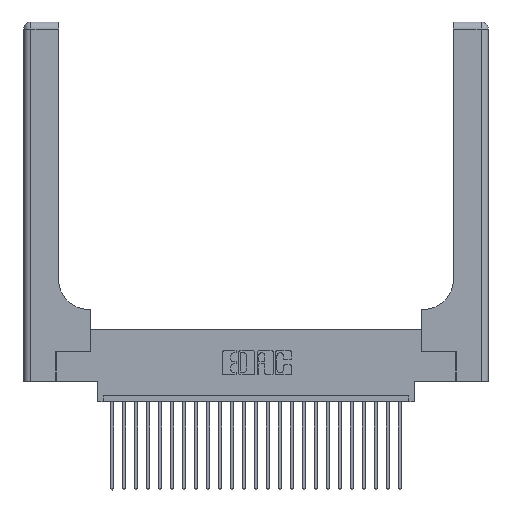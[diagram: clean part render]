
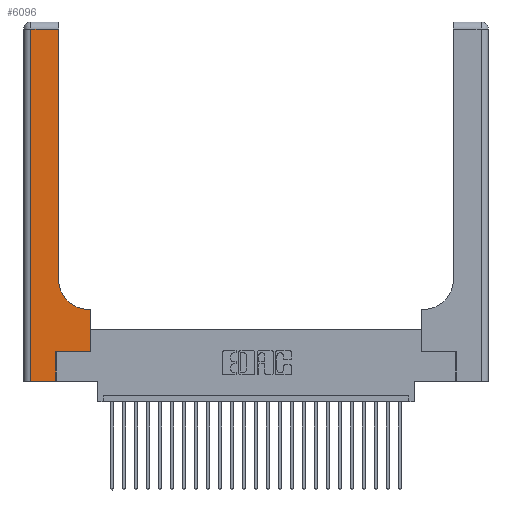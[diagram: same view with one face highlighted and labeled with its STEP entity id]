
A CAD part, top view. The second image highlights one B-rep face of the part: STEP entity #6096.
In plain terms, the highlighted planar face has unit normal (0, 0, 1).
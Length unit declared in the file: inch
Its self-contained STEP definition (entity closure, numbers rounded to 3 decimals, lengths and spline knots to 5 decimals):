
#202 = CARTESIAN_POINT ( 'NONE',  ( 0.269, 0.25, 0.37 ) ) ;
#352 = CARTESIAN_POINT ( 'NONE',  ( 0.2915, 0.6, 0.37 ) ) ;
#2135 = DIRECTION ( 'NONE',  ( -1., 0., 0. ) ) ;
#2240 = DIRECTION ( 'NONE',  ( 1., 0., 0. ) ) ;
#2931 = DIRECTION ( 'NONE',  ( 0., 1., 0. ) ) ;
#3102 = CARTESIAN_POINT ( 'NONE',  ( 0.269, 0., 0.37 ) ) ;
#3140 = EDGE_CURVE ( 'NONE', #15892, #25523, #5019, .T. ) ;
#3253 = DIRECTION ( 'NONE',  ( 0., 1., 0. ) ) ;
#4117 = VERTEX_POINT ( 'NONE', #5091 ) ;
#4272 = EDGE_CURVE ( 'NONE', #12906, #7709, #6530, .T. ) ;
#4456 = CARTESIAN_POINT ( 'NONE',  ( 0.5415, 0.85, 0.37 ) ) ;
#5019 = LINE ( 'NONE', #15736, #18499 ) ;
#5091 = CARTESIAN_POINT ( 'NONE',  ( 0.06, 2.94, 0.37 ) ) ;
#5233 = VECTOR ( 'NONE', #12712, 39.37008 ) ;
#5398 = LINE ( 'NONE', #202, #12792 ) ;
#5425 = EDGE_CURVE ( 'NONE', #25523, #17110, #17441, .T. ) ;
#5749 = DIRECTION ( 'NONE',  ( 0., 1., 0. ) ) ;
#5812 = ORIENTED_EDGE ( 'NONE', *, *, #4272, .T. ) ;
#6096 = ADVANCED_FACE ( 'NONE', ( #8397 ), #20490, .F. ) ;
#6505 = ORIENTED_EDGE ( 'NONE', *, *, #19280, .T. ) ;
#6530 = LINE ( 'NONE', #3102, #16541 ) ;
#6579 = EDGE_CURVE ( 'NONE', #17346, #4117, #7742, .T. ) ;
#6978 = EDGE_CURVE ( 'NONE', #4117, #7243, #22437, .T. ) ;
#7023 = AXIS2_PLACEMENT_3D ( 'NONE', #16443, #26383, #8324 ) ;
#7243 = VERTEX_POINT ( 'NONE', #25869 ) ;
#7392 = VECTOR ( 'NONE', #22353, 39.37008 ) ;
#7709 = VERTEX_POINT ( 'NONE', #20073 ) ;
#7742 = LINE ( 'NONE', #18617, #13545 ) ;
#8054 = CARTESIAN_POINT ( 'NONE',  ( 0.269, 0., 0.37 ) ) ;
#8059 = VECTOR ( 'NONE', #3253, 39.37008 ) ;
#8324 = DIRECTION ( 'NONE',  ( -1., 0., 0. ) ) ;
#8397 = FACE_OUTER_BOUND ( 'NONE', #21916, .T. ) ;
#8559 = EDGE_CURVE ( 'NONE', #7709, #15892, #5398, .T. ) ;
#8919 = EDGE_CURVE ( 'NONE', #7243, #12906, #10067, .T. ) ;
#10067 = LINE ( 'NONE', #24749, #21543 ) ;
#10941 = ORIENTED_EDGE ( 'NONE', *, *, #8559, .T. ) ;
#11507 = CARTESIAN_POINT ( 'NONE',  ( 0.2915, 3., 0.37 ) ) ;
#12445 = AXIS2_PLACEMENT_3D ( 'NONE', #4456, #16676, #22934 ) ;
#12712 = DIRECTION ( 'NONE',  ( -1., 0., 0. ) ) ;
#12792 = VECTOR ( 'NONE', #2240, 39.37008 ) ;
#12906 = VERTEX_POINT ( 'NONE', #8054 ) ;
#13545 = VECTOR ( 'NONE', #2135, 39.37008 ) ;
#14787 = EDGE_CURVE ( 'NONE', #15656, #17346, #18959, .T. ) ;
#14878 = ORIENTED_EDGE ( 'NONE', *, *, #6978, .T. ) ;
#15656 = VERTEX_POINT ( 'NONE', #19767 ) ;
#15736 = CARTESIAN_POINT ( 'NONE',  ( 0.5585, 0.25, 0.37 ) ) ;
#15892 = VERTEX_POINT ( 'NONE', #18965 ) ;
#16423 = CARTESIAN_POINT ( 'NONE',  ( 0.06, 3., 0.37 ) ) ;
#16443 = CARTESIAN_POINT ( 'NONE',  ( 0., 3., 0.37 ) ) ;
#16541 = VECTOR ( 'NONE', #2931, 39.37008 ) ;
#16676 = DIRECTION ( 'NONE',  ( 0., 0., -1. ) ) ;
#17110 = VERTEX_POINT ( 'NONE', #17229 ) ;
#17229 = CARTESIAN_POINT ( 'NONE',  ( 0.5415, 0.6, 0.37 ) ) ;
#17346 = VERTEX_POINT ( 'NONE', #19593 ) ;
#17441 = LINE ( 'NONE', #352, #5233 ) ;
#18499 = VECTOR ( 'NONE', #5749, 39.37008 ) ;
#18565 = CARTESIAN_POINT ( 'NONE',  ( 0.5585, 0.6, 0.37 ) ) ;
#18617 = CARTESIAN_POINT ( 'NONE',  ( 0., 2.94, 0.37 ) ) ;
#18959 = LINE ( 'NONE', #11507, #8059 ) ;
#18965 = CARTESIAN_POINT ( 'NONE',  ( 0.5585, 0.25, 0.37 ) ) ;
#19280 = EDGE_CURVE ( 'NONE', #17110, #15656, #23455, .T. ) ;
#19593 = CARTESIAN_POINT ( 'NONE',  ( 0.2915, 2.94, 0.37 ) ) ;
#19767 = CARTESIAN_POINT ( 'NONE',  ( 0.2915, 0.85, 0.37 ) ) ;
#20073 = CARTESIAN_POINT ( 'NONE',  ( 0.269, 0.25, 0.37 ) ) ;
#20427 = ORIENTED_EDGE ( 'NONE', *, *, #5425, .T. ) ;
#20490 = PLANE ( 'NONE',  #7023 ) ;
#20572 = ORIENTED_EDGE ( 'NONE', *, *, #8919, .T. ) ;
#21543 = VECTOR ( 'NONE', #22959, 39.37008 ) ;
#21916 = EDGE_LOOP ( 'NONE', ( #22742, #22339, #14878, #20572, #5812, #10941, #24985, #20427, #6505 ) ) ;
#22339 = ORIENTED_EDGE ( 'NONE', *, *, #6579, .T. ) ;
#22353 = DIRECTION ( 'NONE',  ( 0., -1., 0. ) ) ;
#22437 = LINE ( 'NONE', #16423, #7392 ) ;
#22742 = ORIENTED_EDGE ( 'NONE', *, *, #14787, .T. ) ;
#22934 = DIRECTION ( 'NONE',  ( 1., 0., 0. ) ) ;
#22959 = DIRECTION ( 'NONE',  ( 1., 0., 0. ) ) ;
#23455 = CIRCLE ( 'NONE', #12445, 0.25 ) ;
#24749 = CARTESIAN_POINT ( 'NONE',  ( 0., 0., 0.37 ) ) ;
#24985 = ORIENTED_EDGE ( 'NONE', *, *, #3140, .T. ) ;
#25523 = VERTEX_POINT ( 'NONE', #18565 ) ;
#25869 = CARTESIAN_POINT ( 'NONE',  ( 0.06, 0., 0.37 ) ) ;
#26383 = DIRECTION ( 'NONE',  ( 0., 0., -1. ) ) ;
